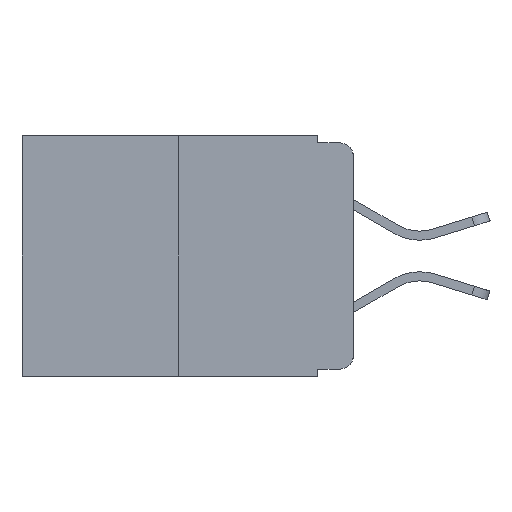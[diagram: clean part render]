
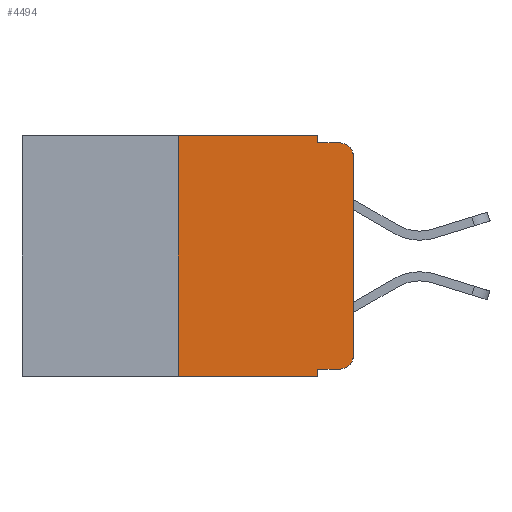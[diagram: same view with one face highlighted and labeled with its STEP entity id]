
A CAD part, left-side view. The second image highlights one B-rep face of the part: STEP entity #4494.
In plain terms, the highlighted planar face has unit normal (-1, 0, 0).
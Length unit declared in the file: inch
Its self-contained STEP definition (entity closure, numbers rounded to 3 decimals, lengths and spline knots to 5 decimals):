
#424 = EDGE_CURVE ( 'NONE', #12254, #7794, #21326, .T. ) ;
#449 = CARTESIAN_POINT ( 'NONE',  ( 0., 0.051, 0. ) ) ;
#1334 = CIRCLE ( 'NONE', #9006, 0.02 ) ;
#1360 = DIRECTION ( 'NONE',  ( 0., -1., 0. ) ) ;
#1429 = VECTOR ( 'NONE', #18526, 39.37008 ) ;
#1717 = VERTEX_POINT ( 'NONE', #15912 ) ;
#1772 = VECTOR ( 'NONE', #22142, 39.37008 ) ;
#1773 = EDGE_CURVE ( 'NONE', #1717, #11131, #13617, .T. ) ;
#2306 = CARTESIAN_POINT ( 'NONE',  ( 0., 0., -0.313 ) ) ;
#2383 = LINE ( 'NONE', #10832, #1772 ) ;
#2406 = DIRECTION ( 'NONE',  ( 0., 0., 1. ) ) ;
#3077 = EDGE_CURVE ( 'NONE', #15298, #11043, #6192, .T. ) ;
#3238 = DIRECTION ( 'NONE',  ( 0., -1., 0. ) ) ;
#3353 = VERTEX_POINT ( 'NONE', #15170 ) ;
#3394 = CARTESIAN_POINT ( 'NONE',  ( 0., 0.051, -0.01 ) ) ;
#3908 = ORIENTED_EDGE ( 'NONE', *, *, #22829, .T. ) ;
#4076 = CARTESIAN_POINT ( 'NONE',  ( 0., 0.02, -0.313 ) ) ;
#4494 = ADVANCED_FACE ( 'NONE', ( #4599 ), #21943, .F. ) ;
#4497 = CARTESIAN_POINT ( 'NONE',  ( 0., 0.25, -0.343 ) ) ;
#4599 = FACE_OUTER_BOUND ( 'NONE', #15389, .T. ) ;
#4798 = CARTESIAN_POINT ( 'NONE',  ( 0., 0.473, 0. ) ) ;
#4851 = ORIENTED_EDGE ( 'NONE', *, *, #1773, .F. ) ;
#5730 = EDGE_CURVE ( 'NONE', #15298, #7258, #2383, .T. ) ;
#5769 = CARTESIAN_POINT ( 'NONE',  ( 0., 0.25, 0. ) ) ;
#6059 = DIRECTION ( 'NONE',  ( 0., 0., -1. ) ) ;
#6192 = LINE ( 'NONE', #19832, #15299 ) ;
#6383 = CARTESIAN_POINT ( 'NONE',  ( 0., 0.02, -0.01 ) ) ;
#6448 = EDGE_CURVE ( 'NONE', #7794, #1717, #6667, .T. ) ;
#6512 = ORIENTED_EDGE ( 'NONE', *, *, #3077, .T. ) ;
#6667 = LINE ( 'NONE', #8828, #1429 ) ;
#6974 = CARTESIAN_POINT ( 'NONE',  ( 0., 0.051, -0.01 ) ) ;
#7219 = CARTESIAN_POINT ( 'NONE',  ( 0., 0.473, -0.343 ) ) ;
#7258 = VERTEX_POINT ( 'NONE', #23901 ) ;
#7794 = VERTEX_POINT ( 'NONE', #8309 ) ;
#8309 = CARTESIAN_POINT ( 'NONE',  ( 0., 0.25, 0. ) ) ;
#8361 = EDGE_CURVE ( 'NONE', #11043, #21399, #1334, .T. ) ;
#8740 = DIRECTION ( 'NONE',  ( 0., 0., -1. ) ) ;
#8828 = CARTESIAN_POINT ( 'NONE',  ( 0., 0.473, 0. ) ) ;
#8867 = VECTOR ( 'NONE', #3238, 39.37008 ) ;
#8882 = ORIENTED_EDGE ( 'NONE', *, *, #9327, .T. ) ;
#9006 = AXIS2_PLACEMENT_3D ( 'NONE', #4076, #17599, #6059 ) ;
#9327 = EDGE_CURVE ( 'NONE', #12254, #7258, #9493, .T. ) ;
#9493 = LINE ( 'NONE', #7219, #8867 ) ;
#9655 = CARTESIAN_POINT ( 'NONE',  ( 0., 0.02, -0.03 ) ) ;
#10832 = CARTESIAN_POINT ( 'NONE',  ( 0., 0.051, 0. ) ) ;
#11043 = VERTEX_POINT ( 'NONE', #21888 ) ;
#11131 = VERTEX_POINT ( 'NONE', #6974 ) ;
#11610 = DIRECTION ( 'NONE',  ( 0., 0., -1. ) ) ;
#12254 = VERTEX_POINT ( 'NONE', #4497 ) ;
#12331 = DIRECTION ( 'NONE',  ( 0., -1., 0. ) ) ;
#12343 = CARTESIAN_POINT ( 'NONE',  ( 0., 0.051, -0.333 ) ) ;
#13275 = CIRCLE ( 'NONE', #13612, 0.02 ) ;
#13612 = AXIS2_PLACEMENT_3D ( 'NONE', #9655, #22886, #11610 ) ;
#13617 = LINE ( 'NONE', #449, #22417 ) ;
#14403 = ORIENTED_EDGE ( 'NONE', *, *, #5730, .F. ) ;
#14627 = ORIENTED_EDGE ( 'NONE', *, *, #6448, .F. ) ;
#15170 = CARTESIAN_POINT ( 'NONE',  ( 0., 0., -0.03 ) ) ;
#15298 = VERTEX_POINT ( 'NONE', #12343 ) ;
#15299 = VECTOR ( 'NONE', #12331, 39.37008 ) ;
#15389 = EDGE_LOOP ( 'NONE', ( #16692, #3908, #24812, #4851, #14627, #22242, #8882, #14403, #6512, #22329 ) ) ;
#15912 = CARTESIAN_POINT ( 'NONE',  ( 0., 0.051, 0. ) ) ;
#16692 = ORIENTED_EDGE ( 'NONE', *, *, #20335, .T. ) ;
#17460 = AXIS2_PLACEMENT_3D ( 'NONE', #4798, #20165, #8740 ) ;
#17557 = VECTOR ( 'NONE', #23765, 39.37008 ) ;
#17599 = DIRECTION ( 'NONE',  ( -1., 0., 0. ) ) ;
#17676 = LINE ( 'NONE', #3394, #22039 ) ;
#17928 = DIRECTION ( 'NONE',  ( 0., 0., -1. ) ) ;
#18131 = LINE ( 'NONE', #18150, #17557 ) ;
#18150 = CARTESIAN_POINT ( 'NONE',  ( 0., 0., 0. ) ) ;
#18526 = DIRECTION ( 'NONE',  ( 0., -1., 0. ) ) ;
#18871 = VERTEX_POINT ( 'NONE', #6383 ) ;
#19832 = CARTESIAN_POINT ( 'NONE',  ( 0., 0.051, -0.333 ) ) ;
#20165 = DIRECTION ( 'NONE',  ( 1., 0., 0. ) ) ;
#20335 = EDGE_CURVE ( 'NONE', #21399, #3353, #18131, .T. ) ;
#20744 = VECTOR ( 'NONE', #2406, 39.37008 ) ;
#21326 = LINE ( 'NONE', #5769, #20744 ) ;
#21399 = VERTEX_POINT ( 'NONE', #2306 ) ;
#21888 = CARTESIAN_POINT ( 'NONE',  ( 0., 0.02, -0.333 ) ) ;
#21943 = PLANE ( 'NONE',  #17460 ) ;
#22039 = VECTOR ( 'NONE', #1360, 39.37008 ) ;
#22142 = DIRECTION ( 'NONE',  ( 0., 0., -1. ) ) ;
#22242 = ORIENTED_EDGE ( 'NONE', *, *, #424, .F. ) ;
#22329 = ORIENTED_EDGE ( 'NONE', *, *, #8361, .T. ) ;
#22417 = VECTOR ( 'NONE', #17928, 39.37008 ) ;
#22829 = EDGE_CURVE ( 'NONE', #3353, #18871, #13275, .T. ) ;
#22886 = DIRECTION ( 'NONE',  ( -1., 0., 0. ) ) ;
#23765 = DIRECTION ( 'NONE',  ( 0., 0., 1. ) ) ;
#23901 = CARTESIAN_POINT ( 'NONE',  ( 0., 0.051, -0.343 ) ) ;
#24062 = EDGE_CURVE ( 'NONE', #11131, #18871, #17676, .T. ) ;
#24812 = ORIENTED_EDGE ( 'NONE', *, *, #24062, .F. ) ;
